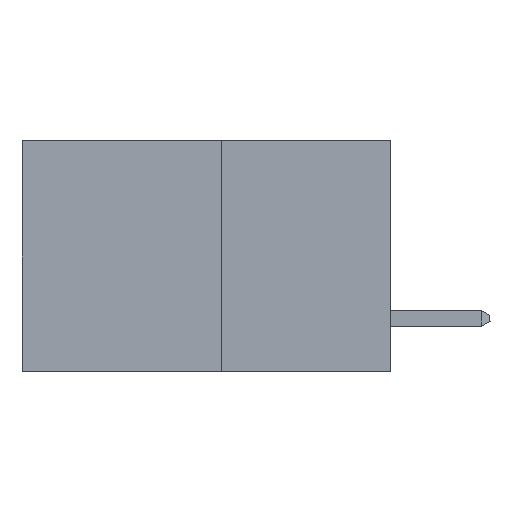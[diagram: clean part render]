
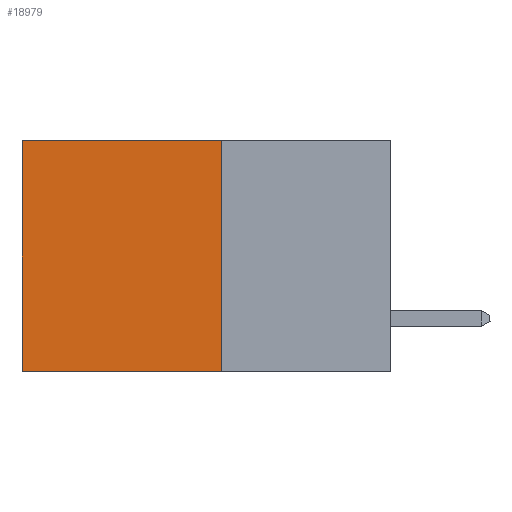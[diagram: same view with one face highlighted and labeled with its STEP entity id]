
A CAD part, left-side view. The second image highlights one B-rep face of the part: STEP entity #18979.
In plain terms, the highlighted planar face has unit normal (-1, 0, 0).
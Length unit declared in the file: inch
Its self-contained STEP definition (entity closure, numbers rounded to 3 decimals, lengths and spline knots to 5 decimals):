
#925 = EDGE_LOOP ( 'NONE', ( #25178, #32093, #12954, #14881 ) ) ;
#1306 = LINE ( 'NONE', #28380, #20372 ) ;
#1634 = CARTESIAN_POINT ( 'NONE',  ( 0.277, 0.59, -0.37 ) ) ;
#2970 = EDGE_CURVE ( 'NONE', #14287, #8474, #28167, .T. ) ;
#4094 = VECTOR ( 'NONE', #33302, 39.37008 ) ;
#4690 = EDGE_CURVE ( 'NONE', #24379, #14287, #1306, .T. ) ;
#5231 = EDGE_CURVE ( 'NONE', #24379, #13175, #19517, .T. ) ;
#7761 = VECTOR ( 'NONE', #33344, 39.37008 ) ;
#8474 = VERTEX_POINT ( 'NONE', #11886 ) ;
#9803 = CARTESIAN_POINT ( 'NONE',  ( 0.277, 0.27, -0.37 ) ) ;
#9965 = VECTOR ( 'NONE', #24974, 39.37008 ) ;
#10401 = DIRECTION ( 'NONE',  ( 0., 1., 0. ) ) ;
#11886 = CARTESIAN_POINT ( 'NONE',  ( 0.277, 0.59, -0.37 ) ) ;
#12954 = ORIENTED_EDGE ( 'NONE', *, *, #5231, .F. ) ;
#13175 = VERTEX_POINT ( 'NONE', #32347 ) ;
#14287 = VERTEX_POINT ( 'NONE', #17545 ) ;
#14795 = CARTESIAN_POINT ( 'NONE',  ( 0.277, 0.27, 0. ) ) ;
#14881 = ORIENTED_EDGE ( 'NONE', *, *, #4690, .T. ) ;
#15008 = DIRECTION ( 'NONE',  ( 1., 0., 0. ) ) ;
#15800 = FACE_OUTER_BOUND ( 'NONE', #925, .T. ) ;
#17545 = CARTESIAN_POINT ( 'NONE',  ( 0.277, 0.59, 0. ) ) ;
#18979 = ADVANCED_FACE ( 'NONE', ( #15800 ), #22707, .F. ) ;
#19517 = LINE ( 'NONE', #30698, #4094 ) ;
#20372 = VECTOR ( 'NONE', #10401, 39.37008 ) ;
#21421 = AXIS2_PLACEMENT_3D ( 'NONE', #9803, #15008, #33055 ) ;
#22707 = PLANE ( 'NONE',  #21421 ) ;
#23114 = CARTESIAN_POINT ( 'NONE',  ( 0.277, 0.27, -0.37 ) ) ;
#24379 = VERTEX_POINT ( 'NONE', #14795 ) ;
#24974 = DIRECTION ( 'NONE',  ( 0., 0., -1. ) ) ;
#25178 = ORIENTED_EDGE ( 'NONE', *, *, #2970, .T. ) ;
#28167 = LINE ( 'NONE', #1634, #9965 ) ;
#28380 = CARTESIAN_POINT ( 'NONE',  ( 0.277, 0.27, 0. ) ) ;
#28395 = LINE ( 'NONE', #23114, #7761 ) ;
#30698 = CARTESIAN_POINT ( 'NONE',  ( 0.277, 0.27, -0.37 ) ) ;
#32006 = EDGE_CURVE ( 'NONE', #13175, #8474, #28395, .T. ) ;
#32093 = ORIENTED_EDGE ( 'NONE', *, *, #32006, .F. ) ;
#32347 = CARTESIAN_POINT ( 'NONE',  ( 0.277, 0.27, -0.37 ) ) ;
#33055 = DIRECTION ( 'NONE',  ( 0., 0., -1. ) ) ;
#33302 = DIRECTION ( 'NONE',  ( 0., 0., -1. ) ) ;
#33344 = DIRECTION ( 'NONE',  ( 0., 1., 0. ) ) ;
